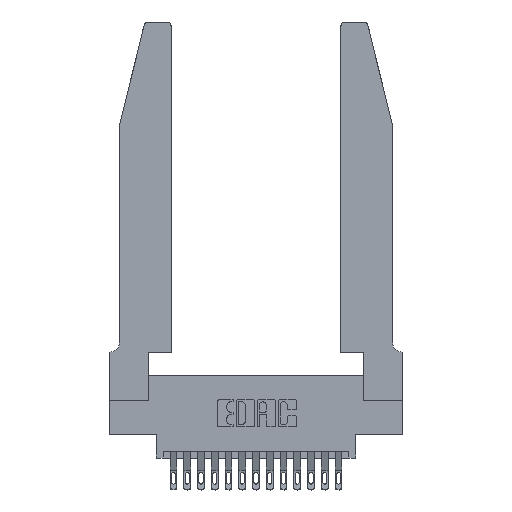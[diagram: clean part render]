
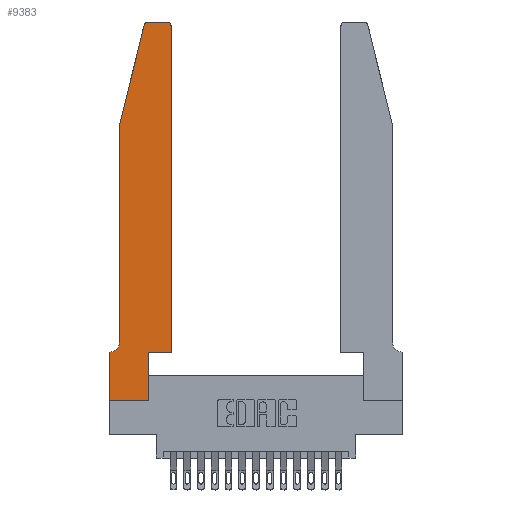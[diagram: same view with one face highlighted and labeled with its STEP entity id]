
A CAD part, top view. The second image highlights one B-rep face of the part: STEP entity #9383.
In plain terms, the highlighted planar face has unit normal (0, 0, 1).
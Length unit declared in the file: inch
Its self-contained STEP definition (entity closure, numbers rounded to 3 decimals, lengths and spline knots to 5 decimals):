
#221 = CARTESIAN_POINT ( 'NONE',  ( 0., 0., 0.37 ) ) ;
#244 = VECTOR ( 'NONE', #16937, 39.37008 ) ;
#454 = CARTESIAN_POINT ( 'NONE',  ( 0.0755, 0.42, 0.37 ) ) ;
#1019 = DIRECTION ( 'NONE',  ( 1., 0., 0. ) ) ;
#1194 = CARTESIAN_POINT ( 'NONE',  ( 0.4205, 2.72, 0.37 ) ) ;
#1578 = ORIENTED_EDGE ( 'NONE', *, *, #17169, .T. ) ;
#1811 = CIRCLE ( 'NONE', #10057, 0.03 ) ;
#2145 = DIRECTION ( 'NONE',  ( 0., -1., 0. ) ) ;
#2285 = CARTESIAN_POINT ( 'NONE',  ( 0., 0.35, 0.37 ) ) ;
#2358 = CARTESIAN_POINT ( 'NONE',  ( 0.2865, 0., 0.37 ) ) ;
#2665 = VERTEX_POINT ( 'NONE', #454 ) ;
#2680 = ORIENTED_EDGE ( 'NONE', *, *, #10921, .T. ) ;
#2754 = DIRECTION ( 'NONE',  ( 0., 0., -1. ) ) ;
#2831 = DIRECTION ( 'NONE',  ( 1., 0., 0. ) ) ;
#3183 = VERTEX_POINT ( 'NONE', #3474 ) ;
#3474 = CARTESIAN_POINT ( 'NONE',  ( 0.25487, 2.72718, 0.37 ) ) ;
#3767 = CIRCLE ( 'NONE', #8962, 0.07 ) ;
#3828 = DIRECTION ( 'NONE',  ( 0., 0., 1. ) ) ;
#3910 = ORIENTED_EDGE ( 'NONE', *, *, #10206, .T. ) ;
#3931 = VERTEX_POINT ( 'NONE', #2358 ) ;
#3974 = VECTOR ( 'NONE', #10596, 39.37008 ) ;
#4101 = VECTOR ( 'NONE', #17153, 39.37008 ) ;
#4194 = ORIENTED_EDGE ( 'NONE', *, *, #16391, .T. ) ;
#4457 = LINE ( 'NONE', #6690, #244 ) ;
#4751 = EDGE_CURVE ( 'NONE', #11609, #5135, #6412, .T. ) ;
#4909 = CARTESIAN_POINT ( 'NONE',  ( 0.0755, 2., 0.37 ) ) ;
#5135 = VERTEX_POINT ( 'NONE', #8140 ) ;
#5396 = CARTESIAN_POINT ( 'NONE',  ( 0.0755, 0.35, 0.37 ) ) ;
#5586 = CARTESIAN_POINT ( 'NONE',  ( 0.284, 2.72, 0.37 ) ) ;
#5920 = CARTESIAN_POINT ( 'NONE',  ( 0.4505, 0.35, 0.37 ) ) ;
#6306 = VECTOR ( 'NONE', #13778, 39.37008 ) ;
#6412 = CIRCLE ( 'NONE', #13272, 0.03 ) ;
#6664 = VECTOR ( 'NONE', #7342, 39.37008 ) ;
#6690 = CARTESIAN_POINT ( 'NONE',  ( 0.0755, 2., 0.37 ) ) ;
#6724 = EDGE_CURVE ( 'NONE', #19234, #3183, #1811, .T. ) ;
#7087 = DIRECTION ( 'NONE',  ( 1., 0., 0. ) ) ;
#7342 = DIRECTION ( 'NONE',  ( 0., 1., 0. ) ) ;
#7916 = ORIENTED_EDGE ( 'NONE', *, *, #18022, .T. ) ;
#7945 = EDGE_CURVE ( 'NONE', #17627, #16963, #9769, .T. ) ;
#8011 = LINE ( 'NONE', #221, #19236 ) ;
#8140 = CARTESIAN_POINT ( 'NONE',  ( 0.4205, 2.75, 0.37 ) ) ;
#8396 = EDGE_CURVE ( 'NONE', #15530, #13723, #9320, .T. ) ;
#8631 = ORIENTED_EDGE ( 'NONE', *, *, #7945, .T. ) ;
#8799 = ORIENTED_EDGE ( 'NONE', *, *, #11563, .T. ) ;
#8962 = AXIS2_PLACEMENT_3D ( 'NONE', #11655, #2754, #13139 ) ;
#9273 = CARTESIAN_POINT ( 'NONE',  ( 0.284, 2.75, 0.37 ) ) ;
#9320 = LINE ( 'NONE', #9728, #13236 ) ;
#9383 = ADVANCED_FACE ( 'NONE', ( #15215 ), #11228, .T. ) ;
#9597 = LINE ( 'NONE', #5920, #13071 ) ;
#9617 = EDGE_CURVE ( 'NONE', #16963, #11609, #9597, .T. ) ;
#9728 = CARTESIAN_POINT ( 'NONE',  ( 0., 0., 0.37 ) ) ;
#9769 = LINE ( 'NONE', #18808, #13258 ) ;
#10057 = AXIS2_PLACEMENT_3D ( 'NONE', #5586, #15860, #7087 ) ;
#10206 = EDGE_CURVE ( 'NONE', #2665, #12074, #3767, .T. ) ;
#10384 = DIRECTION ( 'NONE',  ( 0., 1., 0. ) ) ;
#10596 = DIRECTION ( 'NONE',  ( -1., 0., 0. ) ) ;
#10862 = ORIENTED_EDGE ( 'NONE', *, *, #6724, .T. ) ;
#10921 = EDGE_CURVE ( 'NONE', #5135, #19234, #19153, .T. ) ;
#11228 = PLANE ( 'NONE',  #16885 ) ;
#11425 = CARTESIAN_POINT ( 'NONE',  ( 0.0755, 2., 0.37 ) ) ;
#11563 = EDGE_CURVE ( 'NONE', #3183, #18236, #4457, .T. ) ;
#11609 = VERTEX_POINT ( 'NONE', #17063 ) ;
#11655 = CARTESIAN_POINT ( 'NONE',  ( 0.0055, 0.42, 0.37 ) ) ;
#11725 = DIRECTION ( 'NONE',  ( 0., 0., 1. ) ) ;
#11977 = EDGE_CURVE ( 'NONE', #18236, #2665, #17535, .T. ) ;
#12074 = VERTEX_POINT ( 'NONE', #16984 ) ;
#13071 = VECTOR ( 'NONE', #10384, 39.37008 ) ;
#13139 = DIRECTION ( 'NONE',  ( -1., 0., 0. ) ) ;
#13236 = VECTOR ( 'NONE', #2145, 39.37008 ) ;
#13258 = VECTOR ( 'NONE', #1019, 39.37008 ) ;
#13272 = AXIS2_PLACEMENT_3D ( 'NONE', #1194, #11725, #2831 ) ;
#13723 = VERTEX_POINT ( 'NONE', #13896 ) ;
#13778 = DIRECTION ( 'NONE',  ( 0., -1., 0. ) ) ;
#13896 = CARTESIAN_POINT ( 'NONE',  ( 0., 0., 0.37 ) ) ;
#14166 = CARTESIAN_POINT ( 'NONE',  ( 0.4505, 0.35, 0.37 ) ) ;
#14179 = DIRECTION ( 'NONE',  ( 1., 0., 0. ) ) ;
#14672 = CARTESIAN_POINT ( 'NONE',  ( 0.2865, 0.35, 0.37 ) ) ;
#14969 = ORIENTED_EDGE ( 'NONE', *, *, #8396, .T. ) ;
#15003 = CARTESIAN_POINT ( 'NONE',  ( 0.2605, 2.75, 0.37 ) ) ;
#15215 = FACE_OUTER_BOUND ( 'NONE', #18797, .T. ) ;
#15530 = VERTEX_POINT ( 'NONE', #16477 ) ;
#15860 = DIRECTION ( 'NONE',  ( 0., 0., 1. ) ) ;
#16022 = ORIENTED_EDGE ( 'NONE', *, *, #11977, .T. ) ;
#16308 = LINE ( 'NONE', #5396, #4101 ) ;
#16391 = EDGE_CURVE ( 'NONE', #12074, #15530, #16308, .T. ) ;
#16477 = CARTESIAN_POINT ( 'NONE',  ( 0., 0.35, 0.37 ) ) ;
#16700 = DIRECTION ( 'NONE',  ( 1., 0., 0. ) ) ;
#16885 = AXIS2_PLACEMENT_3D ( 'NONE', #2285, #3828, #14179 ) ;
#16937 = DIRECTION ( 'NONE',  ( -0.239, -0.971, 0. ) ) ;
#16963 = VERTEX_POINT ( 'NONE', #14166 ) ;
#16984 = CARTESIAN_POINT ( 'NONE',  ( 0.0055, 0.35, 0.37 ) ) ;
#17063 = CARTESIAN_POINT ( 'NONE',  ( 0.4505, 2.72, 0.37 ) ) ;
#17153 = DIRECTION ( 'NONE',  ( -1., 0., 0. ) ) ;
#17169 = EDGE_CURVE ( 'NONE', #3931, #17627, #18330, .T. ) ;
#17236 = CARTESIAN_POINT ( 'NONE',  ( 0.2865, 0.35, 0.37 ) ) ;
#17535 = LINE ( 'NONE', #4909, #6306 ) ;
#17627 = VERTEX_POINT ( 'NONE', #17236 ) ;
#18022 = EDGE_CURVE ( 'NONE', #13723, #3931, #8011, .T. ) ;
#18236 = VERTEX_POINT ( 'NONE', #11425 ) ;
#18330 = LINE ( 'NONE', #14672, #6664 ) ;
#18772 = ORIENTED_EDGE ( 'NONE', *, *, #4751, .T. ) ;
#18797 = EDGE_LOOP ( 'NONE', ( #2680, #10862, #8799, #16022, #3910, #4194, #14969, #7916, #1578, #8631, #19199, #18772 ) ) ;
#18808 = CARTESIAN_POINT ( 'NONE',  ( 0.4505, 0.35, 0.37 ) ) ;
#19153 = LINE ( 'NONE', #15003, #3974 ) ;
#19199 = ORIENTED_EDGE ( 'NONE', *, *, #9617, .T. ) ;
#19234 = VERTEX_POINT ( 'NONE', #9273 ) ;
#19236 = VECTOR ( 'NONE', #16700, 39.37008 ) ;
